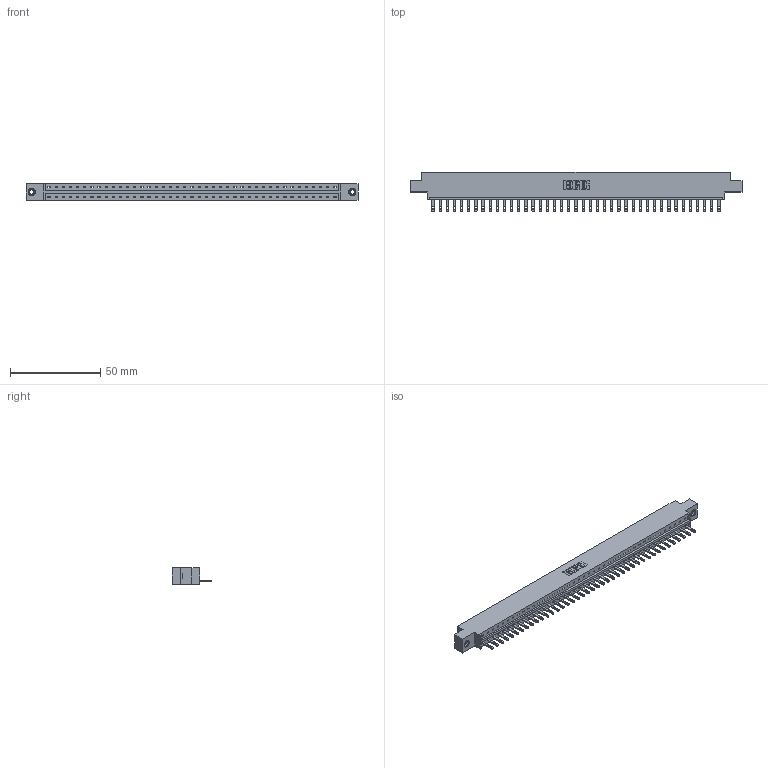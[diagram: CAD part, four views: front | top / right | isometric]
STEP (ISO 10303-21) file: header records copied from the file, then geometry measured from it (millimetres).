
FILE_DESCRIPTION (( 'STEP AP203' ), '1' );
FILE_NAME ('833-041-500-607.STEP', '2020-06-03T18:33:54', ( '' ), ( '' ), 'SwSTEP 2.0', 'SolidWorks 2020', '' );
FILE_SCHEMA (( 'CONFIG_CONTROL_DESIGN' ));
Length unit declared in the file: inch
Products named in the file (4): 345-292-001_345-293-100; 345-250-001_345-250-005-103; 833 Part_Offset - .156 Dia - TI; 833-041-500-607
Assembly tree (44 placements, depth 2):
  833-041-500-607
    833 Part_Offset - .156 Dia - TI
    345-292-001_345-293-100  x41
    345-250-001_345-250-005-103  x2
Bounding box: 184 x 21.85 x 9.4 mm (x, y, z)
Volume: 18290.8 mm3; surface area: 20118.9 mm2
Topology: 44 solids, 44 shells, 2392 faces, 7347 edges, 4890 vertices
Faces by surface type: plane 1582, cylinder 794, cone 12, torus 4
Entity records: 26442 total; most frequent: CARTESIAN_POINT 4544, ORIENTED_EDGE 4514, DIRECTION 3869, EDGE_CURVE 2257, LINE 2105, VECTOR 2105, VERTEX_POINT 1500, AXIS2_PLACEMENT_3D 882
